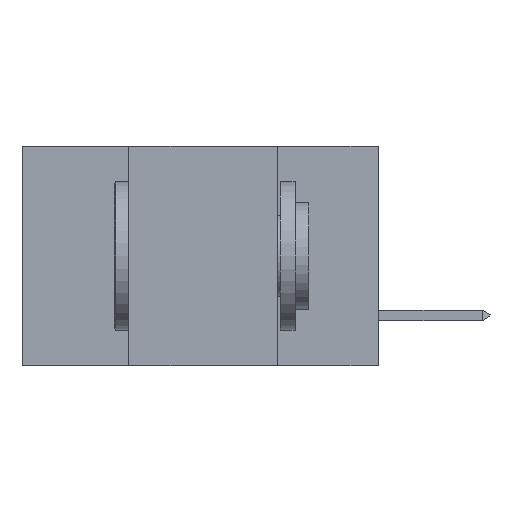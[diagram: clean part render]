
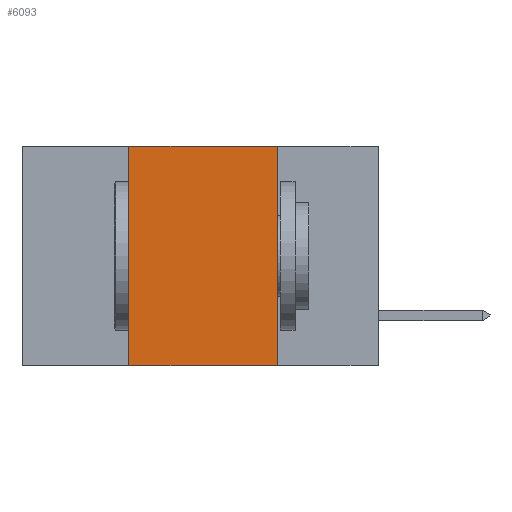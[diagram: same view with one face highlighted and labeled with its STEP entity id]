
A CAD part, left-side view. The second image highlights one B-rep face of the part: STEP entity #6093.
In plain terms, the highlighted planar face has unit normal (-1, 0, 0).
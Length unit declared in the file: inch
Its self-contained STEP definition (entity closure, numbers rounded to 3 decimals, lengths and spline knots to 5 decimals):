
#353 = CARTESIAN_POINT ( 'NONE',  ( 0., 0.6, 0. ) ) ;
#629 = LINE ( 'NONE', #18829, #951 ) ;
#792 = CARTESIAN_POINT ( 'NONE',  ( 0., 0.42, 0. ) ) ;
#951 = VECTOR ( 'NONE', #2257, 39.37008 ) ;
#1049 = DIRECTION ( 'NONE',  ( 0., -1., 0. ) ) ;
#1784 = VERTEX_POINT ( 'NONE', #23945 ) ;
#2119 = EDGE_CURVE ( 'NONE', #2992, #8950, #9790, .T. ) ;
#2257 = DIRECTION ( 'NONE',  ( 0., -1., 0. ) ) ;
#2941 = FACE_OUTER_BOUND ( 'NONE', #27000, .T. ) ;
#2992 = VERTEX_POINT ( 'NONE', #21864 ) ;
#3068 = AXIS2_PLACEMENT_3D ( 'NONE', #353, #13364, #15653 ) ;
#3250 = EDGE_CURVE ( 'NONE', #1784, #19378, #23525, .T. ) ;
#5039 = VECTOR ( 'NONE', #18337, 39.37008 ) ;
#6093 = ADVANCED_FACE ( 'NONE', ( #2941 ), #13460, .F. ) ;
#8593 = LINE ( 'NONE', #9731, #15464 ) ;
#8950 = VERTEX_POINT ( 'NONE', #17026 ) ;
#9731 = CARTESIAN_POINT ( 'NONE',  ( 0., 0.6, 0. ) ) ;
#9790 = LINE ( 'NONE', #13943, #5039 ) ;
#11351 = CARTESIAN_POINT ( 'NONE',  ( 0., 0.42, 0. ) ) ;
#13364 = DIRECTION ( 'NONE',  ( 1., 0., 0. ) ) ;
#13460 = PLANE ( 'NONE',  #3068 ) ;
#13943 = CARTESIAN_POINT ( 'NONE',  ( 0., 0.17, 0. ) ) ;
#15464 = VECTOR ( 'NONE', #1049, 39.37008 ) ;
#15653 = DIRECTION ( 'NONE',  ( 0., 0., -1. ) ) ;
#16050 = EDGE_CURVE ( 'NONE', #1784, #8950, #629, .T. ) ;
#17026 = CARTESIAN_POINT ( 'NONE',  ( 0., 0.17, -0.37 ) ) ;
#18337 = DIRECTION ( 'NONE',  ( 0., 0., -1. ) ) ;
#18829 = CARTESIAN_POINT ( 'NONE',  ( 0., 0.6, -0.37 ) ) ;
#19378 = VERTEX_POINT ( 'NONE', #11351 ) ;
#20511 = ORIENTED_EDGE ( 'NONE', *, *, #3250, .F. ) ;
#20710 = ORIENTED_EDGE ( 'NONE', *, *, #2119, .F. ) ;
#21864 = CARTESIAN_POINT ( 'NONE',  ( 0., 0.17, 0. ) ) ;
#22628 = ORIENTED_EDGE ( 'NONE', *, *, #16050, .T. ) ;
#22830 = DIRECTION ( 'NONE',  ( 0., 0., 1. ) ) ;
#23163 = VECTOR ( 'NONE', #22830, 39.37008 ) ;
#23525 = LINE ( 'NONE', #792, #23163 ) ;
#23945 = CARTESIAN_POINT ( 'NONE',  ( 0., 0.42, -0.37 ) ) ;
#25944 = ORIENTED_EDGE ( 'NONE', *, *, #27711, .F. ) ;
#27000 = EDGE_LOOP ( 'NONE', ( #20710, #25944, #20511, #22628 ) ) ;
#27711 = EDGE_CURVE ( 'NONE', #19378, #2992, #8593, .T. ) ;
